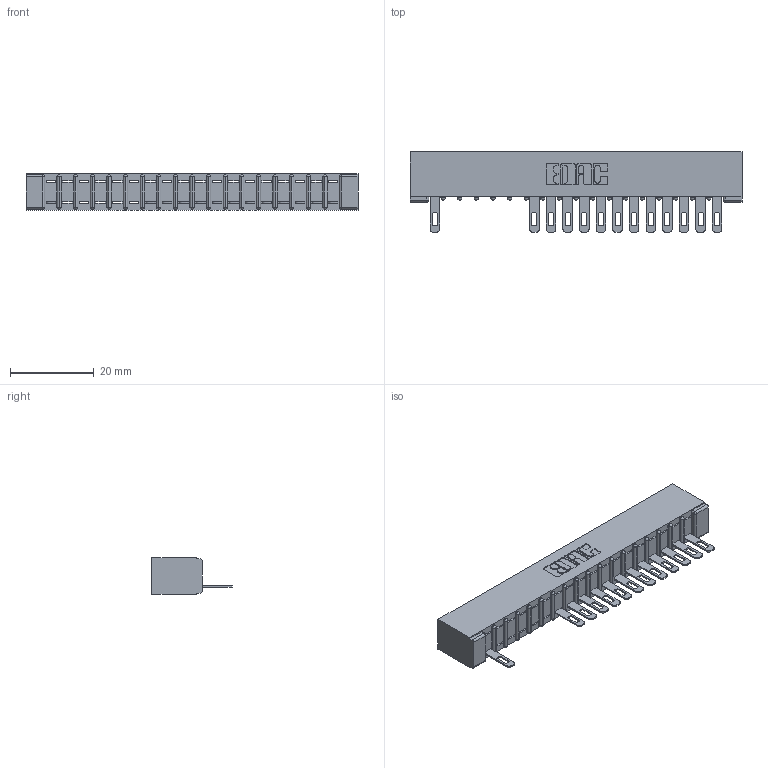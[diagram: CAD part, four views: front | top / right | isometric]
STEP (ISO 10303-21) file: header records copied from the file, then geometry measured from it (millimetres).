
FILE_DESCRIPTION (( 'STEP AP203' ), '1' );
FILE_NAME ('357-018-505-101.STEP', '2018-08-08T04:14:26', ( '' ), ( '' ), 'SwSTEP 2.0', 'SolidWorks 2016', '' );
FILE_SCHEMA (( 'CONFIG_CONTROL_DESIGN' ));
Length unit declared in the file: inch
Products named in the file (3): 307 Part_No Mounting Lugs; 307-290-001_505; 357-018-505-101
Assembly tree (14 placements, depth 2):
  357-018-505-101
    307 Part_No Mounting Lugs
    307-290-001_505  x13
Bounding box: 79.2 x 19.18 x 8.71 mm (x, y, z)
Volume: 5153.9 mm3; surface area: 7817.2 mm2
Topology: 14 solids, 14 shells, 957 faces, 2725 edges, 1746 vertices
Faces by surface type: plane 594, cylinder 325, sphere 38
Entity records: 17926 total; most frequent: CARTESIAN_POINT 3031, ORIENTED_EDGE 3022, DIRECTION 2957, EDGE_CURVE 1511, LINE 1149, VECTOR 1149, VERTEX_POINT 978, AXIS2_PLACEMENT_3D 904
